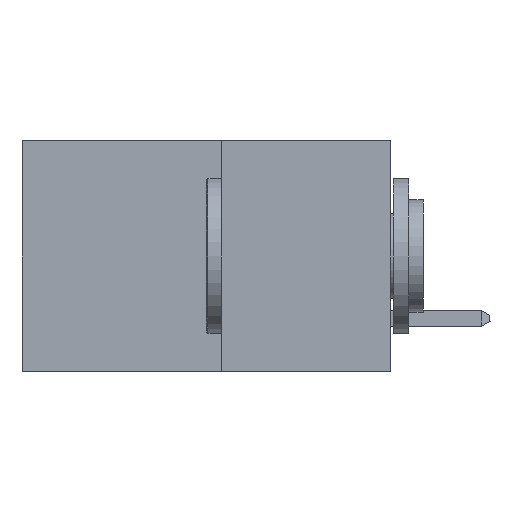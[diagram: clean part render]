
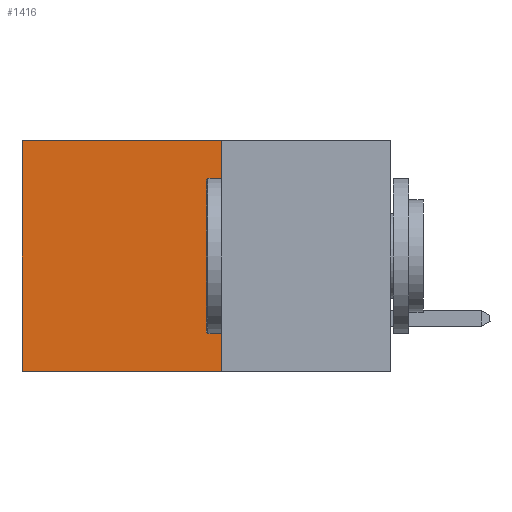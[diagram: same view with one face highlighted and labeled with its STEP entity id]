
A CAD part, left-side view. The second image highlights one B-rep face of the part: STEP entity #1416.
In plain terms, the highlighted planar face has unit normal (-1, 0, 0).
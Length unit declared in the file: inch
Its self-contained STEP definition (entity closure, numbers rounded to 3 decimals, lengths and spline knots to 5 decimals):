
#719 = VERTEX_POINT ( 'NONE', #7099 ) ;
#913 = LINE ( 'NONE', #4299, #1381 ) ;
#1087 = CARTESIAN_POINT ( 'NONE',  ( 0.277, 0.27, -0.37 ) ) ;
#1278 = CARTESIAN_POINT ( 'NONE',  ( 0.277, 0.27, -0.37 ) ) ;
#1381 = VECTOR ( 'NONE', #14516, 39.37008 ) ;
#1416 = ADVANCED_FACE ( 'NONE', ( #10315 ), #17447, .F. ) ;
#3313 = LINE ( 'NONE', #5971, #14510 ) ;
#3817 = ORIENTED_EDGE ( 'NONE', *, *, #15903, .T. ) ;
#4299 = CARTESIAN_POINT ( 'NONE',  ( 0.277, 0.27, 0. ) ) ;
#4534 = EDGE_CURVE ( 'NONE', #7607, #15368, #14484, .T. ) ;
#4804 = EDGE_LOOP ( 'NONE', ( #3817, #9993, #15303, #7410 ) ) ;
#4920 = DIRECTION ( 'NONE',  ( 0., 0., -1. ) ) ;
#5971 = CARTESIAN_POINT ( 'NONE',  ( 0.277, 0.59, -0.37 ) ) ;
#6194 = LINE ( 'NONE', #1278, #17014 ) ;
#6271 = VERTEX_POINT ( 'NONE', #8252 ) ;
#7099 = CARTESIAN_POINT ( 'NONE',  ( 0.277, 0.59, 0. ) ) ;
#7410 = ORIENTED_EDGE ( 'NONE', *, *, #14107, .T. ) ;
#7607 = VERTEX_POINT ( 'NONE', #9004 ) ;
#8252 = CARTESIAN_POINT ( 'NONE',  ( 0.277, 0.59, -0.37 ) ) ;
#8571 = DIRECTION ( 'NONE',  ( 0., 1., 0. ) ) ;
#8912 = DIRECTION ( 'NONE',  ( 0., 0., -1. ) ) ;
#9004 = CARTESIAN_POINT ( 'NONE',  ( 0.277, 0.27, 0. ) ) ;
#9993 = ORIENTED_EDGE ( 'NONE', *, *, #18326, .F. ) ;
#10315 = FACE_OUTER_BOUND ( 'NONE', #4804, .T. ) ;
#12140 = DIRECTION ( 'NONE',  ( 0., 0., -1. ) ) ;
#12144 = CARTESIAN_POINT ( 'NONE',  ( 0.277, 0.27, -0.37 ) ) ;
#14107 = EDGE_CURVE ( 'NONE', #7607, #719, #913, .T. ) ;
#14484 = LINE ( 'NONE', #12144, #16603 ) ;
#14489 = DIRECTION ( 'NONE',  ( 1., 0., 0. ) ) ;
#14510 = VECTOR ( 'NONE', #8912, 39.37008 ) ;
#14516 = DIRECTION ( 'NONE',  ( 0., 1., 0. ) ) ;
#15116 = CARTESIAN_POINT ( 'NONE',  ( 0.277, 0.27, -0.37 ) ) ;
#15303 = ORIENTED_EDGE ( 'NONE', *, *, #4534, .F. ) ;
#15368 = VERTEX_POINT ( 'NONE', #1087 ) ;
#15903 = EDGE_CURVE ( 'NONE', #719, #6271, #3313, .T. ) ;
#16603 = VECTOR ( 'NONE', #12140, 39.37008 ) ;
#17014 = VECTOR ( 'NONE', #8571, 39.37008 ) ;
#17447 = PLANE ( 'NONE',  #17656 ) ;
#17656 = AXIS2_PLACEMENT_3D ( 'NONE', #15116, #14489, #4920 ) ;
#18326 = EDGE_CURVE ( 'NONE', #15368, #6271, #6194, .T. ) ;
